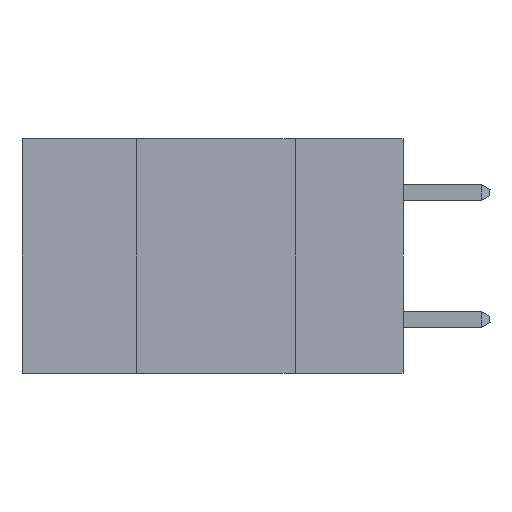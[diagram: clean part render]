
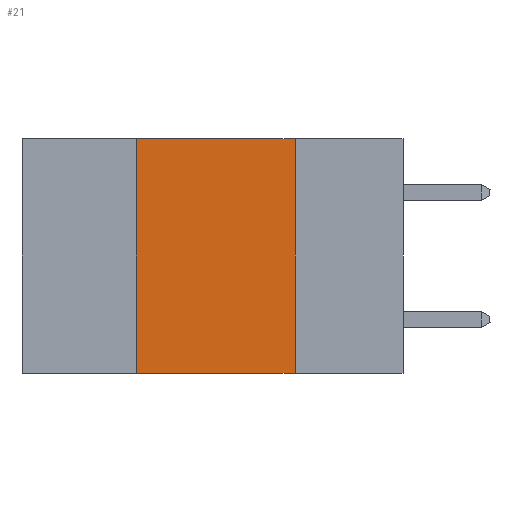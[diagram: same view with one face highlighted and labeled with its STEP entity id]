
A CAD part, left-side view. The second image highlights one B-rep face of the part: STEP entity #21.
In plain terms, the highlighted planar face has unit normal (-1, 0, 0).
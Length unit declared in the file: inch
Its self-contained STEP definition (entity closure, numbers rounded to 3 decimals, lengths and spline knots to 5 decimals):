
#21 = ADVANCED_FACE ( 'NONE', ( #10812 ), #10476, .F. ) ;
#831 = DIRECTION ( 'NONE',  ( 0., 0., 1. ) ) ;
#1269 = ORIENTED_EDGE ( 'NONE', *, *, #14025, .F. ) ;
#1956 = VERTEX_POINT ( 'NONE', #6674 ) ;
#3576 = EDGE_CURVE ( 'NONE', #9510, #1956, #6992, .T. ) ;
#4138 = ORIENTED_EDGE ( 'NONE', *, *, #5018, .F. ) ;
#5018 = EDGE_CURVE ( 'NONE', #15137, #9510, #12341, .T. ) ;
#5417 = VECTOR ( 'NONE', #6481, 39.37008 ) ;
#5496 = CARTESIAN_POINT ( 'NONE',  ( 0., 0.6, 0. ) ) ;
#6481 = DIRECTION ( 'NONE',  ( 0., -1., 0. ) ) ;
#6674 = CARTESIAN_POINT ( 'NONE',  ( 0., 0.17, -0.37 ) ) ;
#6988 = CARTESIAN_POINT ( 'NONE',  ( 0., 0.6, 0. ) ) ;
#6992 = LINE ( 'NONE', #8117, #13211 ) ;
#7661 = AXIS2_PLACEMENT_3D ( 'NONE', #5496, #10493, #10777 ) ;
#7950 = VECTOR ( 'NONE', #14895, 39.37008 ) ;
#8117 = CARTESIAN_POINT ( 'NONE',  ( 0., 0.17, 0. ) ) ;
#9252 = LINE ( 'NONE', #14342, #5417 ) ;
#9425 = DIRECTION ( 'NONE',  ( 0., 0., -1. ) ) ;
#9510 = VERTEX_POINT ( 'NONE', #10831 ) ;
#10476 = PLANE ( 'NONE',  #7661 ) ;
#10493 = DIRECTION ( 'NONE',  ( 1., 0., 0. ) ) ;
#10777 = DIRECTION ( 'NONE',  ( 0., 0., -1. ) ) ;
#10812 = FACE_OUTER_BOUND ( 'NONE', #12548, .T. ) ;
#10831 = CARTESIAN_POINT ( 'NONE',  ( 0., 0.17, 0. ) ) ;
#11839 = VECTOR ( 'NONE', #831, 39.37008 ) ;
#11869 = EDGE_CURVE ( 'NONE', #14543, #1956, #9252, .T. ) ;
#12341 = LINE ( 'NONE', #6988, #7950 ) ;
#12548 = EDGE_LOOP ( 'NONE', ( #15921, #4138, #1269, #13381 ) ) ;
#13211 = VECTOR ( 'NONE', #9425, 39.37008 ) ;
#13381 = ORIENTED_EDGE ( 'NONE', *, *, #11869, .T. ) ;
#13424 = CARTESIAN_POINT ( 'NONE',  ( 0., 0.42, 0. ) ) ;
#13890 = CARTESIAN_POINT ( 'NONE',  ( 0., 0.42, 0. ) ) ;
#14025 = EDGE_CURVE ( 'NONE', #14543, #15137, #15216, .T. ) ;
#14342 = CARTESIAN_POINT ( 'NONE',  ( 0., 0.6, -0.37 ) ) ;
#14543 = VERTEX_POINT ( 'NONE', #16194 ) ;
#14895 = DIRECTION ( 'NONE',  ( 0., -1., 0. ) ) ;
#15137 = VERTEX_POINT ( 'NONE', #13424 ) ;
#15216 = LINE ( 'NONE', #13890, #11839 ) ;
#15921 = ORIENTED_EDGE ( 'NONE', *, *, #3576, .F. ) ;
#16194 = CARTESIAN_POINT ( 'NONE',  ( 0., 0.42, -0.37 ) ) ;
